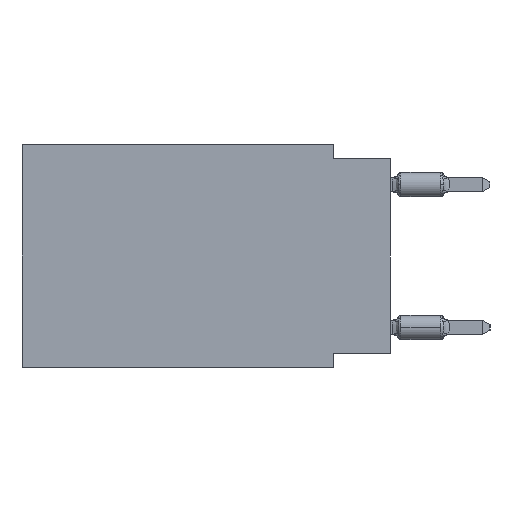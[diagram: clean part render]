
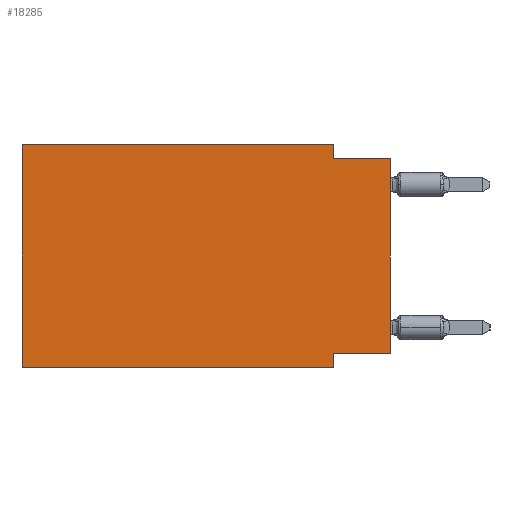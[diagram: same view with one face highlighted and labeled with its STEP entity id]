
A CAD part, left-side view. The second image highlights one B-rep face of the part: STEP entity #18285.
In plain terms, the highlighted planar face has unit normal (-1, 0, 0).
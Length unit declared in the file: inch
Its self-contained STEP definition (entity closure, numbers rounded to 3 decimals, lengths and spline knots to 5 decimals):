
#373 = VECTOR ( 'NONE', #50178, 39.37008 ) ;
#1618 = EDGE_CURVE ( 'NONE', #12551, #15339, #50709, .T. ) ;
#2139 = DIRECTION ( 'NONE',  ( 0., -1., 0. ) ) ;
#3806 = CARTESIAN_POINT ( 'NONE',  ( 0., 0.645, 0. ) ) ;
#4199 = DIRECTION ( 'NONE',  ( 0., 1., 0. ) ) ;
#4774 = DIRECTION ( 'NONE',  ( 0., -1., 0. ) ) ;
#5686 = VERTEX_POINT ( 'NONE', #33452 ) ;
#6842 = DIRECTION ( 'NONE',  ( 0., 0., -1. ) ) ;
#8110 = CARTESIAN_POINT ( 'NONE',  ( 0., 0.1, -0.39 ) ) ;
#8231 = LINE ( 'NONE', #24383, #39836 ) ;
#8347 = ORIENTED_EDGE ( 'NONE', *, *, #8603, .F. ) ;
#8603 = EDGE_CURVE ( 'NONE', #5686, #12551, #21547, .T. ) ;
#9131 = DIRECTION ( 'NONE',  ( 0., 0., -1. ) ) ;
#9337 = CARTESIAN_POINT ( 'NONE',  ( 0., 0.645, 0. ) ) ;
#10987 = VECTOR ( 'NONE', #4199, 39.37008 ) ;
#11999 = VERTEX_POINT ( 'NONE', #47826 ) ;
#12089 = CARTESIAN_POINT ( 'NONE',  ( 0., 0., -0.025 ) ) ;
#12100 = VERTEX_POINT ( 'NONE', #48858 ) ;
#12551 = VERTEX_POINT ( 'NONE', #34906 ) ;
#13346 = LINE ( 'NONE', #32700, #40242 ) ;
#13937 = AXIS2_PLACEMENT_3D ( 'NONE', #43158, #35209, #6842 ) ;
#14655 = EDGE_CURVE ( 'NONE', #15339, #50729, #8231, .T. ) ;
#15209 = LINE ( 'NONE', #3806, #38376 ) ;
#15339 = VERTEX_POINT ( 'NONE', #44354 ) ;
#15684 = VECTOR ( 'NONE', #2139, 39.37008 ) ;
#15949 = VERTEX_POINT ( 'NONE', #41354 ) ;
#17064 = ORIENTED_EDGE ( 'NONE', *, *, #1618, .F. ) ;
#17957 = ORIENTED_EDGE ( 'NONE', *, *, #31314, .T. ) ;
#18285 = ADVANCED_FACE ( 'NONE', ( #40245 ), #48442, .F. ) ;
#20208 = EDGE_CURVE ( 'NONE', #24497, #5686, #15209, .T. ) ;
#21547 = LINE ( 'NONE', #9337, #29915 ) ;
#22082 = CARTESIAN_POINT ( 'NONE',  ( 0., 0.1, 0. ) ) ;
#22282 = LINE ( 'NONE', #38459, #15684 ) ;
#22675 = ORIENTED_EDGE ( 'NONE', *, *, #20208, .F. ) ;
#23413 = EDGE_CURVE ( 'NONE', #11999, #12100, #28247, .T. ) ;
#24383 = CARTESIAN_POINT ( 'NONE',  ( 0., 0., -0.025 ) ) ;
#24497 = VERTEX_POINT ( 'NONE', #46904 ) ;
#26504 = ORIENTED_EDGE ( 'NONE', *, *, #43206, .F. ) ;
#28247 = LINE ( 'NONE', #8110, #42467 ) ;
#29915 = VECTOR ( 'NONE', #46201, 39.37008 ) ;
#31115 = DIRECTION ( 'NONE',  ( 0., 0., 1. ) ) ;
#31314 = EDGE_CURVE ( 'NONE', #15949, #50729, #13346, .T. ) ;
#32700 = CARTESIAN_POINT ( 'NONE',  ( 0., 0., 0. ) ) ;
#33452 = CARTESIAN_POINT ( 'NONE',  ( 0., 0.645, 0. ) ) ;
#33486 = DIRECTION ( 'NONE',  ( 0., 0., 1. ) ) ;
#34906 = CARTESIAN_POINT ( 'NONE',  ( 0., 0.1, 0. ) ) ;
#35209 = DIRECTION ( 'NONE',  ( 1., 0., 0. ) ) ;
#35653 = ORIENTED_EDGE ( 'NONE', *, *, #14655, .F. ) ;
#38376 = VECTOR ( 'NONE', #31115, 39.37008 ) ;
#38459 = CARTESIAN_POINT ( 'NONE',  ( 0., 0.645, -0.39 ) ) ;
#39494 = ORIENTED_EDGE ( 'NONE', *, *, #40547, .T. ) ;
#39764 = EDGE_LOOP ( 'NONE', ( #17957, #35653, #17064, #8347, #22675, #39494, #43221, #26504 ) ) ;
#39836 = VECTOR ( 'NONE', #4774, 39.37008 ) ;
#40242 = VECTOR ( 'NONE', #33486, 39.37008 ) ;
#40245 = FACE_OUTER_BOUND ( 'NONE', #39764, .T. ) ;
#40547 = EDGE_CURVE ( 'NONE', #24497, #12100, #22282, .T. ) ;
#41055 = LINE ( 'NONE', #44245, #10987 ) ;
#41354 = CARTESIAN_POINT ( 'NONE',  ( 0., 0., -0.365 ) ) ;
#42467 = VECTOR ( 'NONE', #9131, 39.37008 ) ;
#43158 = CARTESIAN_POINT ( 'NONE',  ( 0., 0.645, 0. ) ) ;
#43206 = EDGE_CURVE ( 'NONE', #15949, #11999, #41055, .T. ) ;
#43221 = ORIENTED_EDGE ( 'NONE', *, *, #23413, .F. ) ;
#44245 = CARTESIAN_POINT ( 'NONE',  ( 0., 0., -0.365 ) ) ;
#44354 = CARTESIAN_POINT ( 'NONE',  ( 0., 0.1, -0.025 ) ) ;
#46201 = DIRECTION ( 'NONE',  ( 0., -1., 0. ) ) ;
#46904 = CARTESIAN_POINT ( 'NONE',  ( 0., 0.645, -0.39 ) ) ;
#47826 = CARTESIAN_POINT ( 'NONE',  ( 0., 0.1, -0.365 ) ) ;
#48442 = PLANE ( 'NONE',  #13937 ) ;
#48858 = CARTESIAN_POINT ( 'NONE',  ( 0., 0.1, -0.39 ) ) ;
#50178 = DIRECTION ( 'NONE',  ( 0., 0., -1. ) ) ;
#50709 = LINE ( 'NONE', #22082, #373 ) ;
#50729 = VERTEX_POINT ( 'NONE', #12089 ) ;
